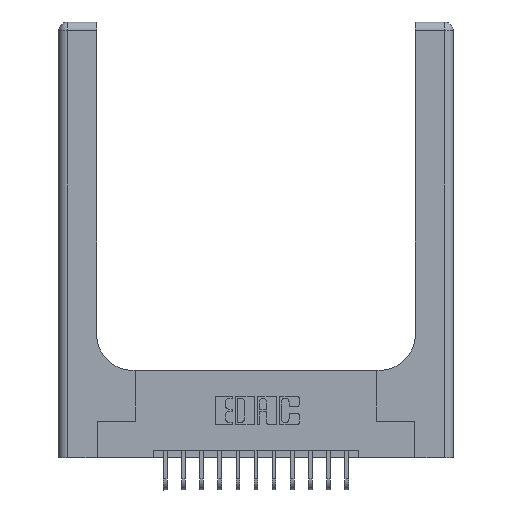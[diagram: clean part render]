
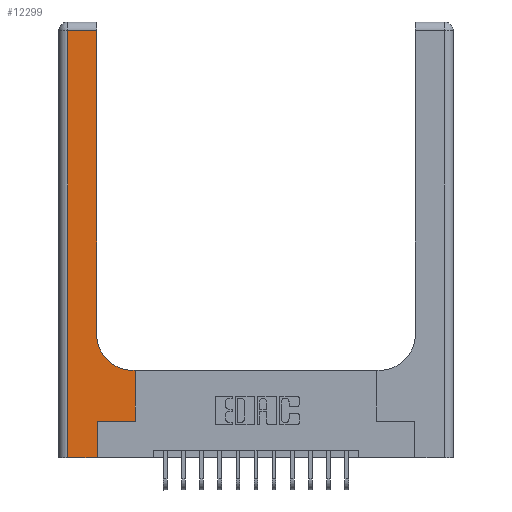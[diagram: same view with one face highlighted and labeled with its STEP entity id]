
A CAD part, top view. The second image highlights one B-rep face of the part: STEP entity #12299.
In plain terms, the highlighted planar face has unit normal (0, 0, 1).
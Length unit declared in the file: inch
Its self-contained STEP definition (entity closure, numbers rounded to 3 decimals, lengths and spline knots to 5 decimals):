
#134 = ORIENTED_EDGE ( 'NONE', *, *, #15009, .T. ) ;
#357 = CARTESIAN_POINT ( 'NONE',  ( 0.265, 0., 0.37 ) ) ;
#435 = ORIENTED_EDGE ( 'NONE', *, *, #16714, .T. ) ;
#530 = DIRECTION ( 'NONE',  ( 1., 0., 0. ) ) ;
#553 = CARTESIAN_POINT ( 'NONE',  ( 0.528, 0.6, 0.37 ) ) ;
#591 = CARTESIAN_POINT ( 'NONE',  ( 0.51, 0.85, 0.37 ) ) ;
#955 = EDGE_CURVE ( 'NONE', #8085, #3379, #1584, .T. ) ;
#1389 = ORIENTED_EDGE ( 'NONE', *, *, #13377, .T. ) ;
#1557 = CARTESIAN_POINT ( 'NONE',  ( 0.528, 0.25, 0.37 ) ) ;
#1567 = CARTESIAN_POINT ( 'NONE',  ( 0.26, 2.94, 0.37 ) ) ;
#1584 = LINE ( 'NONE', #3440, #3583 ) ;
#1653 = CARTESIAN_POINT ( 'NONE',  ( 0.06, 2.94, 0.37 ) ) ;
#1879 = VECTOR ( 'NONE', #8857, 39.37008 ) ;
#2088 = EDGE_CURVE ( 'NONE', #12960, #13324, #6188, .T. ) ;
#2496 = VERTEX_POINT ( 'NONE', #553 ) ;
#2595 = LINE ( 'NONE', #17431, #18321 ) ;
#2668 = ORIENTED_EDGE ( 'NONE', *, *, #3251, .T. ) ;
#3180 = CIRCLE ( 'NONE', #10407, 0.25 ) ;
#3249 = AXIS2_PLACEMENT_3D ( 'NONE', #4987, #7871, #10732 ) ;
#3251 = EDGE_CURVE ( 'NONE', #3379, #12927, #13952, .T. ) ;
#3294 = CARTESIAN_POINT ( 'NONE',  ( 0.51, 0.6, 0.37 ) ) ;
#3379 = VERTEX_POINT ( 'NONE', #14978 ) ;
#3401 = DIRECTION ( 'NONE',  ( 0., 1., 0. ) ) ;
#3440 = CARTESIAN_POINT ( 'NONE',  ( 0., 0., 0.37 ) ) ;
#3559 = LINE ( 'NONE', #13239, #13310 ) ;
#3583 = VECTOR ( 'NONE', #7605, 39.37008 ) ;
#3980 = ORIENTED_EDGE ( 'NONE', *, *, #14371, .T. ) ;
#4511 = LINE ( 'NONE', #1557, #10301 ) ;
#4987 = CARTESIAN_POINT ( 'NONE',  ( 0., 3., 0.37 ) ) ;
#6167 = DIRECTION ( 'NONE',  ( 0., 0., -1. ) ) ;
#6188 = LINE ( 'NONE', #17992, #17929 ) ;
#6277 = LINE ( 'NONE', #11658, #9878 ) ;
#6309 = ORIENTED_EDGE ( 'NONE', *, *, #955, .T. ) ;
#6336 = EDGE_LOOP ( 'NONE', ( #8403, #12222, #3980, #6309, #2668, #1389, #8709, #435, #134 ) ) ;
#6598 = EDGE_CURVE ( 'NONE', #12941, #2496, #4511, .T. ) ;
#7017 = CARTESIAN_POINT ( 'NONE',  ( 0.528, 0.25, 0.37 ) ) ;
#7144 = CARTESIAN_POINT ( 'NONE',  ( 0.265, 0.25, 0.37 ) ) ;
#7261 = DIRECTION ( 'NONE',  ( 0., 1., 0. ) ) ;
#7605 = DIRECTION ( 'NONE',  ( 1., 0., 0. ) ) ;
#7871 = DIRECTION ( 'NONE',  ( 0., 0., -1. ) ) ;
#8085 = VERTEX_POINT ( 'NONE', #13934 ) ;
#8403 = ORIENTED_EDGE ( 'NONE', *, *, #11053, .T. ) ;
#8709 = ORIENTED_EDGE ( 'NONE', *, *, #6598, .T. ) ;
#8818 = DIRECTION ( 'NONE',  ( 0., -1., 0. ) ) ;
#8857 = DIRECTION ( 'NONE',  ( 1., 0., 0. ) ) ;
#8931 = DIRECTION ( 'NONE',  ( -1., 0., 0. ) ) ;
#9878 = VECTOR ( 'NONE', #8818, 39.37008 ) ;
#10209 = VECTOR ( 'NONE', #3401, 39.37008 ) ;
#10301 = VECTOR ( 'NONE', #7261, 39.37008 ) ;
#10407 = AXIS2_PLACEMENT_3D ( 'NONE', #591, #6167, #530 ) ;
#10732 = DIRECTION ( 'NONE',  ( -1., 0., 0. ) ) ;
#11053 = EDGE_CURVE ( 'NONE', #13735, #12960, #2595, .T. ) ;
#11658 = CARTESIAN_POINT ( 'NONE',  ( 0.06, 3., 0.37 ) ) ;
#11682 = FACE_OUTER_BOUND ( 'NONE', #6336, .T. ) ;
#12222 = ORIENTED_EDGE ( 'NONE', *, *, #2088, .T. ) ;
#12299 = ADVANCED_FACE ( 'NONE', ( #11682 ), #17708, .F. ) ;
#12927 = VERTEX_POINT ( 'NONE', #7144 ) ;
#12941 = VERTEX_POINT ( 'NONE', #7017 ) ;
#12960 = VERTEX_POINT ( 'NONE', #1567 ) ;
#13239 = CARTESIAN_POINT ( 'NONE',  ( 0.26, 0.6, 0.37 ) ) ;
#13310 = VECTOR ( 'NONE', #8931, 39.37008 ) ;
#13324 = VERTEX_POINT ( 'NONE', #1653 ) ;
#13377 = EDGE_CURVE ( 'NONE', #12927, #12941, #15826, .T. ) ;
#13597 = DIRECTION ( 'NONE',  ( -1., 0., 0. ) ) ;
#13735 = VERTEX_POINT ( 'NONE', #16808 ) ;
#13934 = CARTESIAN_POINT ( 'NONE',  ( 0.06, 0., 0.37 ) ) ;
#13952 = LINE ( 'NONE', #357, #10209 ) ;
#14371 = EDGE_CURVE ( 'NONE', #13324, #8085, #6277, .T. ) ;
#14481 = CARTESIAN_POINT ( 'NONE',  ( 0.265, 0.25, 0.37 ) ) ;
#14978 = CARTESIAN_POINT ( 'NONE',  ( 0.265, 0., 0.37 ) ) ;
#15009 = EDGE_CURVE ( 'NONE', #17849, #13735, #3180, .T. ) ;
#15826 = LINE ( 'NONE', #14481, #1879 ) ;
#16714 = EDGE_CURVE ( 'NONE', #2496, #17849, #3559, .T. ) ;
#16808 = CARTESIAN_POINT ( 'NONE',  ( 0.26, 0.85, 0.37 ) ) ;
#17431 = CARTESIAN_POINT ( 'NONE',  ( 0.26, 3., 0.37 ) ) ;
#17491 = DIRECTION ( 'NONE',  ( 0., 1., 0. ) ) ;
#17708 = PLANE ( 'NONE',  #3249 ) ;
#17849 = VERTEX_POINT ( 'NONE', #3294 ) ;
#17929 = VECTOR ( 'NONE', #13597, 39.37008 ) ;
#17992 = CARTESIAN_POINT ( 'NONE',  ( 0., 2.94, 0.37 ) ) ;
#18321 = VECTOR ( 'NONE', #17491, 39.37008 ) ;
